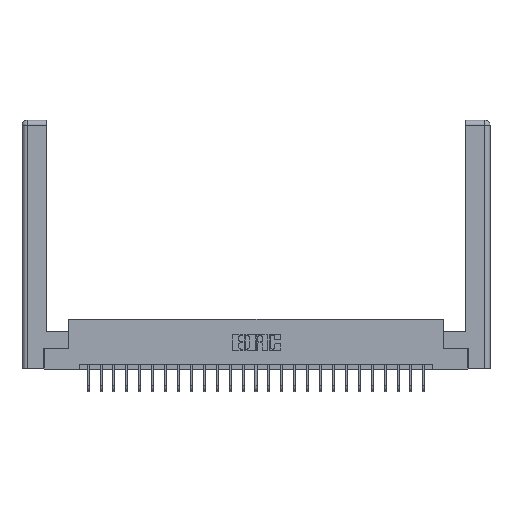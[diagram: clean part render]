
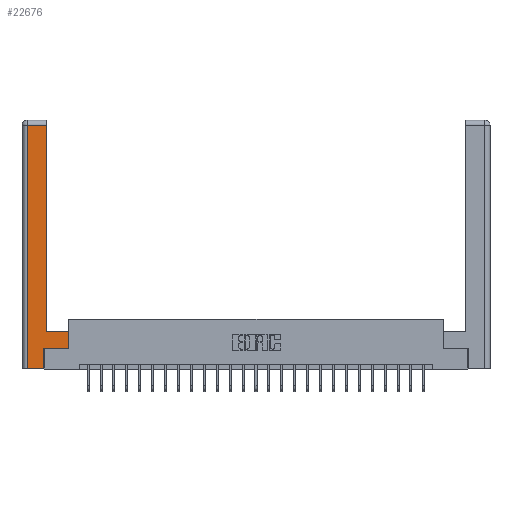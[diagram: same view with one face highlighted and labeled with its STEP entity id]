
A CAD part, top view. The second image highlights one B-rep face of the part: STEP entity #22676.
In plain terms, the highlighted planar face has unit normal (0, 0, 1).
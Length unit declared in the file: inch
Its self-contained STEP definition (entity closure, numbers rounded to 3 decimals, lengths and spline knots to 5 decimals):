
#28 = PLANE ( 'NONE',  #12635 ) ;
#118 = VERTEX_POINT ( 'NONE', #7972 ) ;
#152 = VECTOR ( 'NONE', #7479, 39.37008 ) ;
#441 = DIRECTION ( 'NONE',  ( -1., 0., 0. ) ) ;
#1329 = FACE_OUTER_BOUND ( 'NONE', #6968, .T. ) ;
#1723 = VERTEX_POINT ( 'NONE', #9920 ) ;
#2173 = CARTESIAN_POINT ( 'NONE',  ( 0.265, 0., 0. ) ) ;
#2216 = EDGE_CURVE ( 'NONE', #1723, #2684, #12775, .T. ) ;
#2584 = DIRECTION ( 'NONE',  ( 0., 1., 0. ) ) ;
#2684 = VERTEX_POINT ( 'NONE', #11735 ) ;
#3517 = EDGE_CURVE ( 'NONE', #11363, #118, #17157, .T. ) ;
#4357 = CARTESIAN_POINT ( 'NONE',  ( 0.295, 3., 0. ) ) ;
#5296 = CARTESIAN_POINT ( 'NONE',  ( 0.265, 0.245, 0. ) ) ;
#5846 = DIRECTION ( 'NONE',  ( 0., 0., -1. ) ) ;
#6003 = VERTEX_POINT ( 'NONE', #12749 ) ;
#6452 = CARTESIAN_POINT ( 'NONE',  ( 0.0615, 2.94, 0. ) ) ;
#6642 = VECTOR ( 'NONE', #10900, 39.37008 ) ;
#6660 = CARTESIAN_POINT ( 'NONE',  ( 0.295, 0.45, 0. ) ) ;
#6918 = VECTOR ( 'NONE', #12727, 39.37008 ) ;
#6968 = EDGE_LOOP ( 'NONE', ( #19746, #9041, #11984, #12682, #12196, #24550, #10963, #16722 ) ) ;
#7151 = CARTESIAN_POINT ( 'NONE',  ( 0.565, 0.245, 0. ) ) ;
#7479 = DIRECTION ( 'NONE',  ( 1., 0., 0. ) ) ;
#7972 = CARTESIAN_POINT ( 'NONE',  ( 0.565, 0.245, 0. ) ) ;
#8353 = DIRECTION ( 'NONE',  ( -1., 0., 0. ) ) ;
#8671 = VERTEX_POINT ( 'NONE', #9867 ) ;
#8921 = VECTOR ( 'NONE', #8353, 39.37008 ) ;
#9041 = ORIENTED_EDGE ( 'NONE', *, *, #2216, .T. ) ;
#9867 = CARTESIAN_POINT ( 'NONE',  ( 0.0615, 0., 0. ) ) ;
#9920 = CARTESIAN_POINT ( 'NONE',  ( 0.295, 2.94, 0. ) ) ;
#10374 = VECTOR ( 'NONE', #441, 39.37008 ) ;
#10900 = DIRECTION ( 'NONE',  ( 0., 1., 0. ) ) ;
#10963 = ORIENTED_EDGE ( 'NONE', *, *, #15968, .T. ) ;
#11238 = EDGE_CURVE ( 'NONE', #21499, #11363, #12073, .T. ) ;
#11363 = VERTEX_POINT ( 'NONE', #5296 ) ;
#11735 = CARTESIAN_POINT ( 'NONE',  ( 0.0615, 2.94, 0. ) ) ;
#11984 = ORIENTED_EDGE ( 'NONE', *, *, #24276, .T. ) ;
#12073 = LINE ( 'NONE', #14216, #19228 ) ;
#12086 = DIRECTION ( 'NONE',  ( 0., 1., 0. ) ) ;
#12196 = ORIENTED_EDGE ( 'NONE', *, *, #11238, .T. ) ;
#12635 = AXIS2_PLACEMENT_3D ( 'NONE', #17199, #5846, #19140 ) ;
#12682 = ORIENTED_EDGE ( 'NONE', *, *, #16859, .T. ) ;
#12727 = DIRECTION ( 'NONE',  ( 0., -1., 0. ) ) ;
#12749 = CARTESIAN_POINT ( 'NONE',  ( 0.565, 0.45, 0. ) ) ;
#12775 = LINE ( 'NONE', #6452, #8921 ) ;
#13536 = VERTEX_POINT ( 'NONE', #6660 ) ;
#14216 = CARTESIAN_POINT ( 'NONE',  ( 0.265, 0.245, 0. ) ) ;
#14602 = LINE ( 'NONE', #4357, #16699 ) ;
#15190 = LINE ( 'NONE', #20502, #6642 ) ;
#15968 = EDGE_CURVE ( 'NONE', #118, #6003, #15190, .T. ) ;
#16699 = VECTOR ( 'NONE', #2584, 39.37008 ) ;
#16722 = ORIENTED_EDGE ( 'NONE', *, *, #18657, .T. ) ;
#16859 = EDGE_CURVE ( 'NONE', #8671, #21499, #22680, .T. ) ;
#16958 = EDGE_CURVE ( 'NONE', #13536, #1723, #14602, .T. ) ;
#17157 = LINE ( 'NONE', #7151, #152 ) ;
#17199 = CARTESIAN_POINT ( 'NONE',  ( 0., 0., 0. ) ) ;
#17348 = CARTESIAN_POINT ( 'NONE',  ( 0.295, 0.45, 0. ) ) ;
#17899 = VECTOR ( 'NONE', #21014, 39.37008 ) ;
#18060 = CARTESIAN_POINT ( 'NONE',  ( 0.0615, 0., 0. ) ) ;
#18657 = EDGE_CURVE ( 'NONE', #6003, #13536, #24114, .T. ) ;
#19140 = DIRECTION ( 'NONE',  ( -1., 0., 0. ) ) ;
#19228 = VECTOR ( 'NONE', #12086, 39.37008 ) ;
#19746 = ORIENTED_EDGE ( 'NONE', *, *, #16958, .T. ) ;
#20502 = CARTESIAN_POINT ( 'NONE',  ( 0.565, 0.45, 0. ) ) ;
#21014 = DIRECTION ( 'NONE',  ( 1., 0., 0. ) ) ;
#21499 = VERTEX_POINT ( 'NONE', #21887 ) ;
#21887 = CARTESIAN_POINT ( 'NONE',  ( 0.265, 0., 0. ) ) ;
#22676 = ADVANCED_FACE ( 'NONE', ( #1329 ), #28, .F. ) ;
#22680 = LINE ( 'NONE', #2173, #17899 ) ;
#23583 = LINE ( 'NONE', #18060, #6918 ) ;
#24114 = LINE ( 'NONE', #17348, #10374 ) ;
#24276 = EDGE_CURVE ( 'NONE', #2684, #8671, #23583, .T. ) ;
#24550 = ORIENTED_EDGE ( 'NONE', *, *, #3517, .T. ) ;
